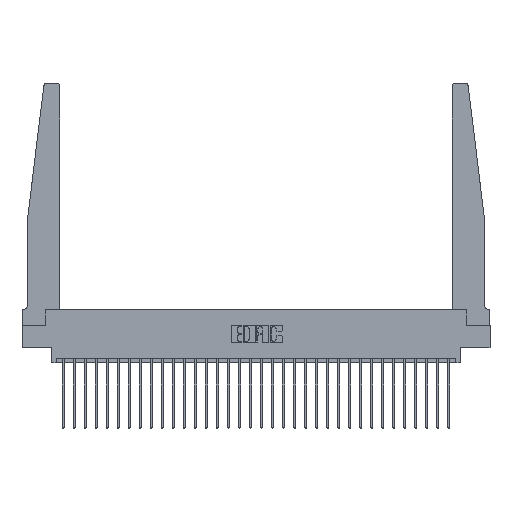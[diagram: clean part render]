
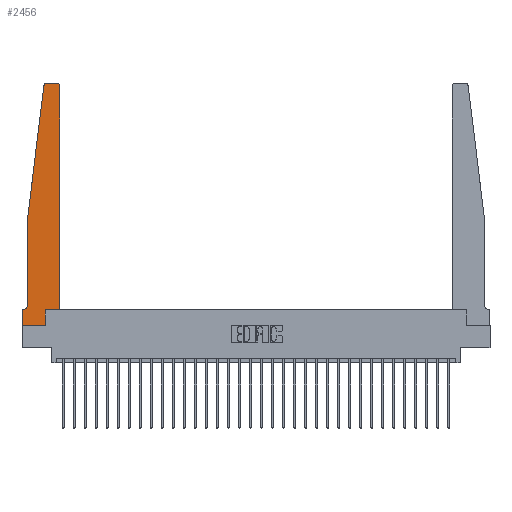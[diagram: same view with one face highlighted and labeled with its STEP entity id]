
A CAD part, top view. The second image highlights one B-rep face of the part: STEP entity #2456.
In plain terms, the highlighted planar face has unit normal (0, 0, 1).
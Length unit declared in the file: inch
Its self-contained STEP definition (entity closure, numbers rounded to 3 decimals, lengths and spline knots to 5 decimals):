
#225 = EDGE_CURVE ( 'NONE', #23204, #26638, #11568, .T. ) ;
#673 = DIRECTION ( 'NONE',  ( 1., 0., 0. ) ) ;
#793 = AXIS2_PLACEMENT_3D ( 'NONE', #11982, #27642, #14256 ) ;
#1496 = CIRCLE ( 'NONE', #793, 0.03 ) ;
#1533 = CARTESIAN_POINT ( 'NONE',  ( 0., 0.1875, 0.37 ) ) ;
#2059 = DIRECTION ( 'NONE',  ( 1., 0., 0. ) ) ;
#2176 = DIRECTION ( 'NONE',  ( 0., 1., 0. ) ) ;
#2456 = ADVANCED_FACE ( 'NONE', ( #4459 ), #15163, .T. ) ;
#3054 = ORIENTED_EDGE ( 'NONE', *, *, #24712, .T. ) ;
#3110 = EDGE_CURVE ( 'NONE', #4910, #11034, #17524, .T. ) ;
#3466 = ORIENTED_EDGE ( 'NONE', *, *, #13841, .T. ) ;
#3845 = DIRECTION ( 'NONE',  ( 1., 0., 0. ) ) ;
#3874 = VERTEX_POINT ( 'NONE', #7987 ) ;
#4101 = VECTOR ( 'NONE', #13909, 39.37008 ) ;
#4144 = CARTESIAN_POINT ( 'NONE',  ( 0.425, 0.18, 0.37 ) ) ;
#4459 = FACE_OUTER_BOUND ( 'NONE', #15132, .T. ) ;
#4868 = CARTESIAN_POINT ( 'NONE',  ( 0.065, 0.1875, 0.37 ) ) ;
#4910 = VERTEX_POINT ( 'NONE', #22007 ) ;
#4924 = VERTEX_POINT ( 'NONE', #27421 ) ;
#5030 = CIRCLE ( 'NONE', #20519, 0.03 ) ;
#5287 = CARTESIAN_POINT ( 'NONE',  ( 0., 0., 0.37 ) ) ;
#5304 = DIRECTION ( 'NONE',  ( 0., 1., 0. ) ) ;
#5807 = VECTOR ( 'NONE', #20681, 39.37008 ) ;
#6427 = VERTEX_POINT ( 'NONE', #24107 ) ;
#6874 = ORIENTED_EDGE ( 'NONE', *, *, #225, .T. ) ;
#6877 = VECTOR ( 'NONE', #673, 39.37008 ) ;
#7111 = CARTESIAN_POINT ( 'NONE',  ( 0.25, 2.75, 0.37 ) ) ;
#7114 = DIRECTION ( 'NONE',  ( -1., 0., 0. ) ) ;
#7270 = EDGE_CURVE ( 'NONE', #21381, #22002, #15228, .T. ) ;
#7458 = CARTESIAN_POINT ( 'NONE',  ( 0.425, 0.18, 0.37 ) ) ;
#7987 = CARTESIAN_POINT ( 'NONE',  ( 0., 0.1875, 0.37 ) ) ;
#8087 = CARTESIAN_POINT ( 'NONE',  ( 0.065, 1.25, 0.37 ) ) ;
#9039 = ORIENTED_EDGE ( 'NONE', *, *, #24319, .T. ) ;
#9563 = CARTESIAN_POINT ( 'NONE',  ( 0.065, 1.25, 0.37 ) ) ;
#9564 = LINE ( 'NONE', #21981, #26084 ) ;
#9672 = VECTOR ( 'NONE', #2176, 39.37008 ) ;
#9805 = EDGE_CURVE ( 'NONE', #25657, #21381, #9564, .T. ) ;
#10195 = EDGE_CURVE ( 'NONE', #6427, #13847, #22214, .T. ) ;
#10259 = VECTOR ( 'NONE', #5304, 39.37008 ) ;
#10754 = CARTESIAN_POINT ( 'NONE',  ( 0.27653, 2.75, 0.37 ) ) ;
#11027 = CARTESIAN_POINT ( 'NONE',  ( 0.015, 0.1875, 0.37 ) ) ;
#11034 = VERTEX_POINT ( 'NONE', #14865 ) ;
#11110 = CARTESIAN_POINT ( 'NONE',  ( 0.015, 0.2375, 0.37 ) ) ;
#11416 = ORIENTED_EDGE ( 'NONE', *, *, #25829, .T. ) ;
#11568 = LINE ( 'NONE', #7111, #4101 ) ;
#11680 = ORIENTED_EDGE ( 'NONE', *, *, #17907, .T. ) ;
#11867 = LINE ( 'NONE', #16087, #5807 ) ;
#11869 = LINE ( 'NONE', #4868, #28576 ) ;
#11914 = ORIENTED_EDGE ( 'NONE', *, *, #3110, .T. ) ;
#11982 = CARTESIAN_POINT ( 'NONE',  ( 0.27653, 2.72, 0.37 ) ) ;
#12542 = CARTESIAN_POINT ( 'NONE',  ( 0.395, 2.75, 0.37 ) ) ;
#13158 = CARTESIAN_POINT ( 'NONE',  ( 0.065, 0.2375, 0.37 ) ) ;
#13407 = DIRECTION ( 'NONE',  ( -1., 0., 0. ) ) ;
#13525 = ORIENTED_EDGE ( 'NONE', *, *, #7270, .T. ) ;
#13841 = EDGE_CURVE ( 'NONE', #3874, #4910, #11867, .T. ) ;
#13847 = VERTEX_POINT ( 'NONE', #22947 ) ;
#13909 = DIRECTION ( 'NONE',  ( -1., 0., 0. ) ) ;
#14256 = DIRECTION ( 'NONE',  ( 1., 0., 0. ) ) ;
#14865 = CARTESIAN_POINT ( 'NONE',  ( 0.2605, 0., 0.37 ) ) ;
#14885 = LINE ( 'NONE', #4144, #21933 ) ;
#15132 = EDGE_LOOP ( 'NONE', ( #6874, #9039, #22856, #19621, #13525, #24394, #3466, #11914, #3054, #11416, #16644, #11680 ) ) ;
#15163 = PLANE ( 'NONE',  #26086 ) ;
#15228 = CIRCLE ( 'NONE', #26337, 0.05 ) ;
#15672 = DIRECTION ( 'NONE',  ( 0., 0., 1. ) ) ;
#15786 = CARTESIAN_POINT ( 'NONE',  ( 0.2605, 0.18, 0.37 ) ) ;
#16087 = CARTESIAN_POINT ( 'NONE',  ( 0., 0., 0.37 ) ) ;
#16644 = ORIENTED_EDGE ( 'NONE', *, *, #10195, .T. ) ;
#17419 = DIRECTION ( 'NONE',  ( 0., 0., 1. ) ) ;
#17524 = LINE ( 'NONE', #5287, #6877 ) ;
#17585 = DIRECTION ( 'NONE',  ( 0., -1., 0. ) ) ;
#17645 = LINE ( 'NONE', #9563, #22191 ) ;
#17907 = EDGE_CURVE ( 'NONE', #13847, #23204, #5030, .T. ) ;
#18093 = EDGE_CURVE ( 'NONE', #22002, #3874, #11869, .T. ) ;
#19621 = ORIENTED_EDGE ( 'NONE', *, *, #9805, .T. ) ;
#20519 = AXIS2_PLACEMENT_3D ( 'NONE', #29057, #15672, #2059 ) ;
#20681 = DIRECTION ( 'NONE',  ( 0., -1., 0. ) ) ;
#20784 = DIRECTION ( 'NONE',  ( -0.122, -0.992, 0. ) ) ;
#20945 = LINE ( 'NONE', #15786, #9672 ) ;
#21279 = CARTESIAN_POINT ( 'NONE',  ( 0.24675, 2.72367, 0.37 ) ) ;
#21381 = VERTEX_POINT ( 'NONE', #13158 ) ;
#21933 = VECTOR ( 'NONE', #26586, 39.37008 ) ;
#21981 = CARTESIAN_POINT ( 'NONE',  ( 0.065, 1.25, 0.37 ) ) ;
#22002 = VERTEX_POINT ( 'NONE', #11027 ) ;
#22007 = CARTESIAN_POINT ( 'NONE',  ( 0., 0., 0.37 ) ) ;
#22191 = VECTOR ( 'NONE', #20784, 39.37008 ) ;
#22214 = LINE ( 'NONE', #7458, #10259 ) ;
#22856 = ORIENTED_EDGE ( 'NONE', *, *, #28196, .T. ) ;
#22947 = CARTESIAN_POINT ( 'NONE',  ( 0.425, 2.72, 0.37 ) ) ;
#23204 = VERTEX_POINT ( 'NONE', #12542 ) ;
#24107 = CARTESIAN_POINT ( 'NONE',  ( 0.425, 0.18, 0.37 ) ) ;
#24319 = EDGE_CURVE ( 'NONE', #26638, #24428, #1496, .T. ) ;
#24394 = ORIENTED_EDGE ( 'NONE', *, *, #18093, .T. ) ;
#24428 = VERTEX_POINT ( 'NONE', #21279 ) ;
#24712 = EDGE_CURVE ( 'NONE', #11034, #4924, #20945, .T. ) ;
#25657 = VERTEX_POINT ( 'NONE', #8087 ) ;
#25829 = EDGE_CURVE ( 'NONE', #4924, #6427, #14885, .T. ) ;
#26084 = VECTOR ( 'NONE', #17585, 39.37008 ) ;
#26086 = AXIS2_PLACEMENT_3D ( 'NONE', #1533, #17419, #3845 ) ;
#26337 = AXIS2_PLACEMENT_3D ( 'NONE', #11110, #26791, #13407 ) ;
#26586 = DIRECTION ( 'NONE',  ( 1., 0., 0. ) ) ;
#26638 = VERTEX_POINT ( 'NONE', #10754 ) ;
#26791 = DIRECTION ( 'NONE',  ( 0., 0., -1. ) ) ;
#27421 = CARTESIAN_POINT ( 'NONE',  ( 0.2605, 0.18, 0.37 ) ) ;
#27642 = DIRECTION ( 'NONE',  ( 0., 0., 1. ) ) ;
#28196 = EDGE_CURVE ( 'NONE', #24428, #25657, #17645, .T. ) ;
#28576 = VECTOR ( 'NONE', #7114, 39.37008 ) ;
#29057 = CARTESIAN_POINT ( 'NONE',  ( 0.395, 2.72, 0.37 ) ) ;
